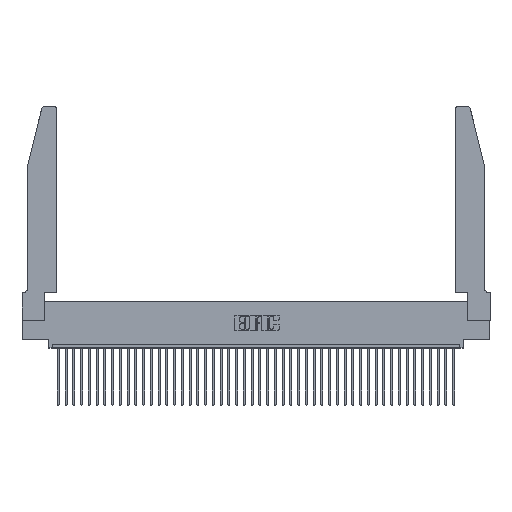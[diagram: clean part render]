
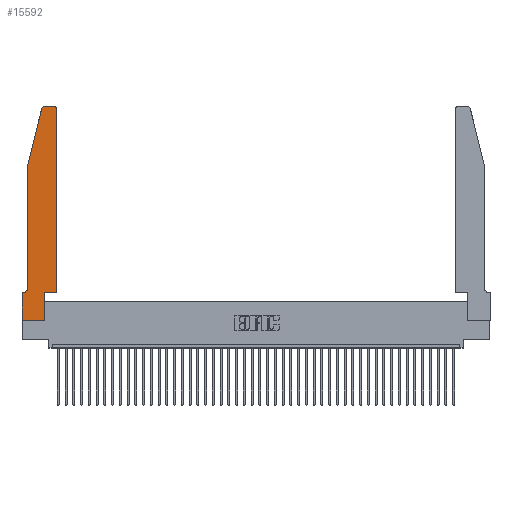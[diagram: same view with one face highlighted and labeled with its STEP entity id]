
A CAD part, top view. The second image highlights one B-rep face of the part: STEP entity #15592.
In plain terms, the highlighted planar face has unit normal (0, 0, 1).
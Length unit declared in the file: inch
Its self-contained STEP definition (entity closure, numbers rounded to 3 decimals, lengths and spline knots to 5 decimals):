
#446 = LINE ( 'NONE', #38771, #35988 ) ;
#1399 = DIRECTION ( 'NONE',  ( 0., -1., 0. ) ) ;
#1496 = LINE ( 'NONE', #20193, #40672 ) ;
#1629 = AXIS2_PLACEMENT_3D ( 'NONE', #8636, #8919, #5538 ) ;
#1766 = VERTEX_POINT ( 'NONE', #37929 ) ;
#1922 = VECTOR ( 'NONE', #31739, 39.37008 ) ;
#2006 = CARTESIAN_POINT ( 'NONE',  ( 0., 0.35, 0.37 ) ) ;
#2575 = LINE ( 'NONE', #18976, #29229 ) ;
#3218 = ORIENTED_EDGE ( 'NONE', *, *, #15342, .T. ) ;
#3332 = VERTEX_POINT ( 'NONE', #20609 ) ;
#3897 = CARTESIAN_POINT ( 'NONE',  ( 0.0055, 0.35, 0.37 ) ) ;
#5003 = LINE ( 'NONE', #31589, #1922 ) ;
#5045 = AXIS2_PLACEMENT_3D ( 'NONE', #9436, #9706, #6325 ) ;
#5538 = DIRECTION ( 'NONE',  ( 1., 0., 0. ) ) ;
#5816 = CIRCLE ( 'NONE', #37957, 0.07 ) ;
#5939 = VECTOR ( 'NONE', #26817, 39.37008 ) ;
#6325 = DIRECTION ( 'NONE',  ( 1., 0., 0. ) ) ;
#6357 = CARTESIAN_POINT ( 'NONE',  ( 0.4505, 0.35, 0.37 ) ) ;
#7120 = LINE ( 'NONE', #8309, #9641 ) ;
#7432 = ORIENTED_EDGE ( 'NONE', *, *, #9180, .T. ) ;
#7652 = CARTESIAN_POINT ( 'NONE',  ( 0.25487, 2.72718, 0.37 ) ) ;
#7714 = EDGE_CURVE ( 'NONE', #18544, #8576, #5003, .T. ) ;
#7904 = VERTEX_POINT ( 'NONE', #30384 ) ;
#8309 = CARTESIAN_POINT ( 'NONE',  ( 0.2605, 2.75, 0.37 ) ) ;
#8334 = ORIENTED_EDGE ( 'NONE', *, *, #32304, .T. ) ;
#8576 = VERTEX_POINT ( 'NONE', #14177 ) ;
#8636 = CARTESIAN_POINT ( 'NONE',  ( 0., 0.35, 0.37 ) ) ;
#8919 = DIRECTION ( 'NONE',  ( 0., 0., 1. ) ) ;
#9180 = EDGE_CURVE ( 'NONE', #8576, #1766, #30568, .T. ) ;
#9285 = LINE ( 'NONE', #29086, #34016 ) ;
#9436 = CARTESIAN_POINT ( 'NONE',  ( 0.284, 2.72, 0.37 ) ) ;
#9641 = VECTOR ( 'NONE', #37470, 39.37008 ) ;
#9706 = DIRECTION ( 'NONE',  ( 0., 0., 1. ) ) ;
#10110 = ORIENTED_EDGE ( 'NONE', *, *, #23999, .T. ) ;
#10396 = DIRECTION ( 'NONE',  ( -1., 0., 0. ) ) ;
#11104 = CARTESIAN_POINT ( 'NONE',  ( 0.0755, 2., 0.37 ) ) ;
#12442 = ORIENTED_EDGE ( 'NONE', *, *, #42050, .T. ) ;
#12473 = EDGE_CURVE ( 'NONE', #33809, #16894, #2575, .T. ) ;
#12852 = VERTEX_POINT ( 'NONE', #3897 ) ;
#13280 = ORIENTED_EDGE ( 'NONE', *, *, #19313, .T. ) ;
#13802 = DIRECTION ( 'NONE',  ( 0., 0., 1. ) ) ;
#14177 = CARTESIAN_POINT ( 'NONE',  ( 0.0755, 2., 0.37 ) ) ;
#15220 = DIRECTION ( 'NONE',  ( 0., 1., 0. ) ) ;
#15342 = EDGE_CURVE ( 'NONE', #36743, #3332, #28588, .T. ) ;
#15592 = ADVANCED_FACE ( 'NONE', ( #27990 ), #31570, .T. ) ;
#16706 = EDGE_LOOP ( 'NONE', ( #38654, #13280, #30614, #7432, #10110, #12442, #8334, #3218, #37368, #22570, #18296, #30135 ) ) ;
#16894 = VERTEX_POINT ( 'NONE', #28373 ) ;
#16963 = DIRECTION ( 'NONE',  ( 0., 0., -1. ) ) ;
#17503 = DIRECTION ( 'NONE',  ( 0., -1., 0. ) ) ;
#18047 = VERTEX_POINT ( 'NONE', #2006 ) ;
#18296 = ORIENTED_EDGE ( 'NONE', *, *, #12473, .T. ) ;
#18544 = VERTEX_POINT ( 'NONE', #7652 ) ;
#18976 = CARTESIAN_POINT ( 'NONE',  ( 0.4505, 0.35, 0.37 ) ) ;
#19313 = EDGE_CURVE ( 'NONE', #22834, #18544, #31356, .T. ) ;
#20086 = EDGE_CURVE ( 'NONE', #16894, #7904, #22154, .T. ) ;
#20165 = CARTESIAN_POINT ( 'NONE',  ( 0., 0., 0.37 ) ) ;
#20193 = CARTESIAN_POINT ( 'NONE',  ( 0.0755, 0.35, 0.37 ) ) ;
#20372 = CARTESIAN_POINT ( 'NONE',  ( 0., 0., 0.37 ) ) ;
#20609 = CARTESIAN_POINT ( 'NONE',  ( 0.2865, 0., 0.37 ) ) ;
#22154 = CIRCLE ( 'NONE', #38727, 0.03 ) ;
#22570 = ORIENTED_EDGE ( 'NONE', *, *, #37805, .T. ) ;
#22574 = CARTESIAN_POINT ( 'NONE',  ( 0., 0., 0.37 ) ) ;
#22834 = VERTEX_POINT ( 'NONE', #34515 ) ;
#22989 = CARTESIAN_POINT ( 'NONE',  ( 0.2865, 0.35, 0.37 ) ) ;
#23052 = DIRECTION ( 'NONE',  ( 1., 0., 0. ) ) ;
#23488 = CARTESIAN_POINT ( 'NONE',  ( 0.4205, 2.72, 0.37 ) ) ;
#23999 = EDGE_CURVE ( 'NONE', #1766, #12852, #5816, .T. ) ;
#26029 = DIRECTION ( 'NONE',  ( 1., 0., 0. ) ) ;
#26817 = DIRECTION ( 'NONE',  ( 1., 0., 0. ) ) ;
#26907 = EDGE_CURVE ( 'NONE', #7904, #22834, #7120, .T. ) ;
#27990 = FACE_OUTER_BOUND ( 'NONE', #16706, .T. ) ;
#28373 = CARTESIAN_POINT ( 'NONE',  ( 0.4505, 2.72, 0.37 ) ) ;
#28588 = LINE ( 'NONE', #20165, #5939 ) ;
#28692 = LINE ( 'NONE', #20372, #31373 ) ;
#29086 = CARTESIAN_POINT ( 'NONE',  ( 0.4505, 0.35, 0.37 ) ) ;
#29229 = VECTOR ( 'NONE', #15220, 39.37008 ) ;
#30135 = ORIENTED_EDGE ( 'NONE', *, *, #20086, .T. ) ;
#30384 = CARTESIAN_POINT ( 'NONE',  ( 0.4205, 2.75, 0.37 ) ) ;
#30568 = LINE ( 'NONE', #11104, #31075 ) ;
#30614 = ORIENTED_EDGE ( 'NONE', *, *, #7714, .T. ) ;
#31075 = VECTOR ( 'NONE', #1399, 39.37008 ) ;
#31356 = CIRCLE ( 'NONE', #5045, 0.03 ) ;
#31373 = VECTOR ( 'NONE', #17503, 39.37008 ) ;
#31570 = PLANE ( 'NONE',  #1629 ) ;
#31589 = CARTESIAN_POINT ( 'NONE',  ( 0.0755, 2., 0.37 ) ) ;
#31739 = DIRECTION ( 'NONE',  ( -0.239, -0.971, 0. ) ) ;
#32049 = EDGE_CURVE ( 'NONE', #3332, #33819, #446, .T. ) ;
#32304 = EDGE_CURVE ( 'NONE', #18047, #36743, #28692, .T. ) ;
#33261 = DIRECTION ( 'NONE',  ( -1., 0., 0. ) ) ;
#33809 = VERTEX_POINT ( 'NONE', #6357 ) ;
#33819 = VERTEX_POINT ( 'NONE', #22989 ) ;
#34016 = VECTOR ( 'NONE', #26029, 39.37008 ) ;
#34515 = CARTESIAN_POINT ( 'NONE',  ( 0.284, 2.75, 0.37 ) ) ;
#35988 = VECTOR ( 'NONE', #42649, 39.37008 ) ;
#36743 = VERTEX_POINT ( 'NONE', #22574 ) ;
#36885 = CARTESIAN_POINT ( 'NONE',  ( 0.0055, 0.42, 0.37 ) ) ;
#37368 = ORIENTED_EDGE ( 'NONE', *, *, #32049, .T. ) ;
#37470 = DIRECTION ( 'NONE',  ( -1., 0., 0. ) ) ;
#37805 = EDGE_CURVE ( 'NONE', #33819, #33809, #9285, .T. ) ;
#37929 = CARTESIAN_POINT ( 'NONE',  ( 0.0755, 0.42, 0.37 ) ) ;
#37957 = AXIS2_PLACEMENT_3D ( 'NONE', #36885, #16963, #33261 ) ;
#38654 = ORIENTED_EDGE ( 'NONE', *, *, #26907, .T. ) ;
#38727 = AXIS2_PLACEMENT_3D ( 'NONE', #23488, #13802, #23052 ) ;
#38771 = CARTESIAN_POINT ( 'NONE',  ( 0.2865, 0.35, 0.37 ) ) ;
#40672 = VECTOR ( 'NONE', #10396, 39.37008 ) ;
#42050 = EDGE_CURVE ( 'NONE', #12852, #18047, #1496, .T. ) ;
#42649 = DIRECTION ( 'NONE',  ( 0., 1., 0. ) ) ;
